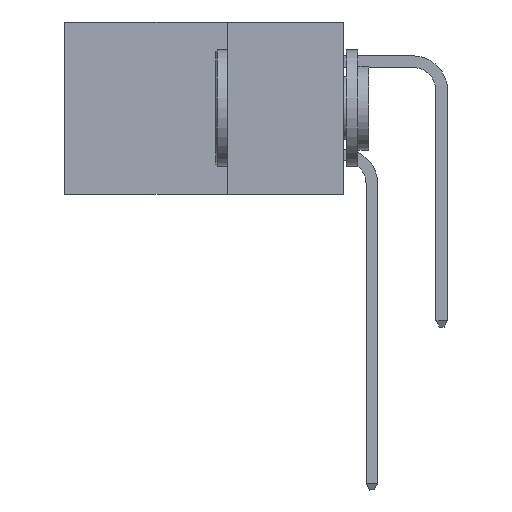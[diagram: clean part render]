
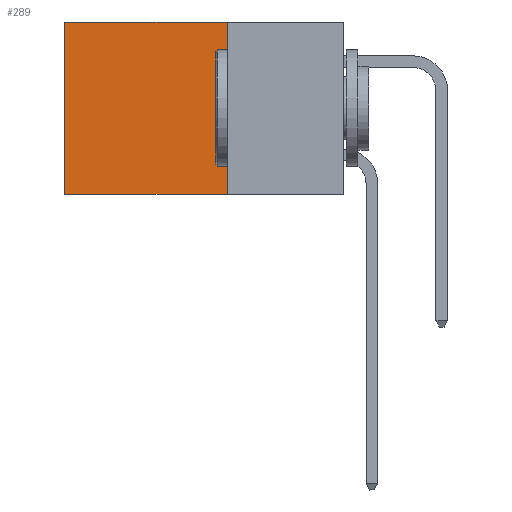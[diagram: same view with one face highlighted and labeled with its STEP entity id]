
A CAD part, left-side view. The second image highlights one B-rep face of the part: STEP entity #289.
In plain terms, the highlighted planar face has unit normal (-1, 0, 0).
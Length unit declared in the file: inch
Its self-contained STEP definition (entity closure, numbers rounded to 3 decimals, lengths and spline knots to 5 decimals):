
#289 = ADVANCED_FACE ( 'NONE', ( #16668 ), #14688, .F. ) ;
#406 = VECTOR ( 'NONE', #26328, 39.37008 ) ;
#981 = EDGE_CURVE ( 'NONE', #27209, #22907, #20981, .T. ) ;
#1697 = ORIENTED_EDGE ( 'NONE', *, *, #9792, .T. ) ;
#4339 = LINE ( 'NONE', #26092, #15188 ) ;
#7295 = LINE ( 'NONE', #10064, #406 ) ;
#9792 = EDGE_CURVE ( 'NONE', #17247, #27209, #7295, .T. ) ;
#9832 = DIRECTION ( 'NONE',  ( 0., 0., -1. ) ) ;
#10064 = CARTESIAN_POINT ( 'NONE',  ( 0.2615, 0.25, 0. ) ) ;
#10111 = AXIS2_PLACEMENT_3D ( 'NONE', #14585, #25892, #23400 ) ;
#11522 = VECTOR ( 'NONE', #16998, 39.37008 ) ;
#13944 = ORIENTED_EDGE ( 'NONE', *, *, #22094, .F. ) ;
#14585 = CARTESIAN_POINT ( 'NONE',  ( 0.2615, 0.25, -0.37 ) ) ;
#14658 = CARTESIAN_POINT ( 'NONE',  ( 0.2615, 0.25, -0.37 ) ) ;
#14688 = PLANE ( 'NONE',  #10111 ) ;
#14792 = VECTOR ( 'NONE', #19165, 39.37008 ) ;
#15188 = VECTOR ( 'NONE', #9832, 39.37008 ) ;
#16668 = FACE_OUTER_BOUND ( 'NONE', #18345, .T. ) ;
#16998 = DIRECTION ( 'NONE',  ( 0., 1., 0. ) ) ;
#17247 = VERTEX_POINT ( 'NONE', #18908 ) ;
#18345 = EDGE_LOOP ( 'NONE', ( #19626, #21540, #13944, #1697 ) ) ;
#18908 = CARTESIAN_POINT ( 'NONE',  ( 0.2615, 0.25, 0. ) ) ;
#19165 = DIRECTION ( 'NONE',  ( 0., 0., -1. ) ) ;
#19626 = ORIENTED_EDGE ( 'NONE', *, *, #981, .T. ) ;
#19904 = CARTESIAN_POINT ( 'NONE',  ( 0.2615, 0.6, -0.37 ) ) ;
#20981 = LINE ( 'NONE', #24731, #14792 ) ;
#21540 = ORIENTED_EDGE ( 'NONE', *, *, #27927, .F. ) ;
#22094 = EDGE_CURVE ( 'NONE', #17247, #25879, #4339, .T. ) ;
#22485 = CARTESIAN_POINT ( 'NONE',  ( 0.2615, 0.6, 0. ) ) ;
#22907 = VERTEX_POINT ( 'NONE', #19904 ) ;
#23400 = DIRECTION ( 'NONE',  ( 0., 0., -1. ) ) ;
#23929 = LINE ( 'NONE', #14658, #11522 ) ;
#24665 = CARTESIAN_POINT ( 'NONE',  ( 0.2615, 0.25, -0.37 ) ) ;
#24731 = CARTESIAN_POINT ( 'NONE',  ( 0.2615, 0.6, -0.37 ) ) ;
#25879 = VERTEX_POINT ( 'NONE', #24665 ) ;
#25892 = DIRECTION ( 'NONE',  ( 1., 0., 0. ) ) ;
#26092 = CARTESIAN_POINT ( 'NONE',  ( 0.2615, 0.25, -0.37 ) ) ;
#26328 = DIRECTION ( 'NONE',  ( 0., 1., 0. ) ) ;
#27209 = VERTEX_POINT ( 'NONE', #22485 ) ;
#27927 = EDGE_CURVE ( 'NONE', #25879, #22907, #23929, .T. ) ;
